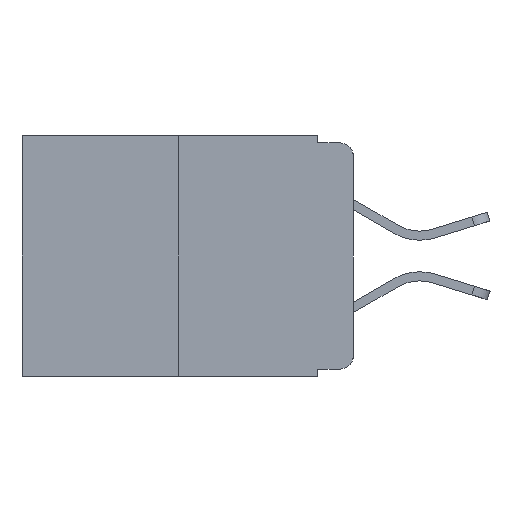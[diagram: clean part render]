
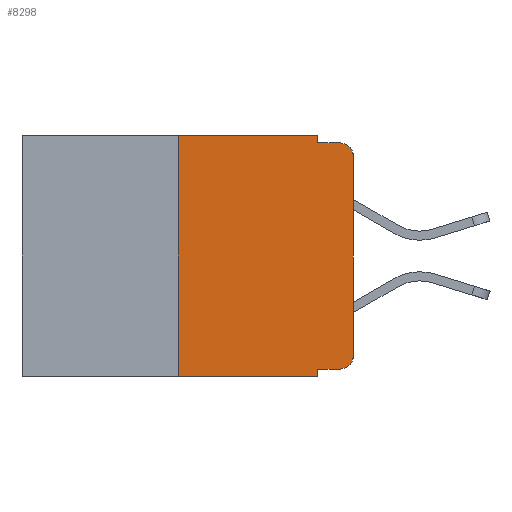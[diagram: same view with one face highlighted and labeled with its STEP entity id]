
A CAD part, left-side view. The second image highlights one B-rep face of the part: STEP entity #8298.
In plain terms, the highlighted planar face has unit normal (-1, 0, 0).
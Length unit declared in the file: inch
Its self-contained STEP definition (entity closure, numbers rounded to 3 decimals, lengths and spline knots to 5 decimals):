
#426 = EDGE_CURVE ( 'NONE', #20141, #12894, #7068, .T. ) ;
#635 = CARTESIAN_POINT ( 'NONE',  ( 0., 0., -0.313 ) ) ;
#849 = LINE ( 'NONE', #15361, #4133 ) ;
#969 = VECTOR ( 'NONE', #13384, 39.37008 ) ;
#1814 = CARTESIAN_POINT ( 'NONE',  ( 0., 0.25, -0.343 ) ) ;
#1913 = EDGE_CURVE ( 'NONE', #13388, #16300, #17655, .T. ) ;
#1970 = CARTESIAN_POINT ( 'NONE',  ( 0., 0.02, -0.313 ) ) ;
#2210 = VERTEX_POINT ( 'NONE', #3482 ) ;
#2233 = VECTOR ( 'NONE', #20647, 39.37008 ) ;
#2246 = LINE ( 'NONE', #18679, #21154 ) ;
#2588 = LINE ( 'NONE', #6047, #2233 ) ;
#2892 = ORIENTED_EDGE ( 'NONE', *, *, #12941, .T. ) ;
#3252 = PLANE ( 'NONE',  #8954 ) ;
#3482 = CARTESIAN_POINT ( 'NONE',  ( 0., 0., -0.03 ) ) ;
#3603 = CARTESIAN_POINT ( 'NONE',  ( 0., 0.051, -0.333 ) ) ;
#4133 = VECTOR ( 'NONE', #9190, 39.37008 ) ;
#4142 = CARTESIAN_POINT ( 'NONE',  ( 0., 0.051, -0.333 ) ) ;
#4661 = DIRECTION ( 'NONE',  ( 0., 0., -1. ) ) ;
#4762 = DIRECTION ( 'NONE',  ( 1., 0., 0. ) ) ;
#4946 = CARTESIAN_POINT ( 'NONE',  ( 0., 0.02, -0.333 ) ) ;
#5320 = EDGE_CURVE ( 'NONE', #16300, #13942, #5418, .T. ) ;
#5418 = CIRCLE ( 'NONE', #11596, 0.02 ) ;
#5475 = LINE ( 'NONE', #12148, #11381 ) ;
#5669 = ORIENTED_EDGE ( 'NONE', *, *, #7285, .F. ) ;
#6047 = CARTESIAN_POINT ( 'NONE',  ( 0., 0.051, 0. ) ) ;
#6206 = VERTEX_POINT ( 'NONE', #10444 ) ;
#7068 = LINE ( 'NONE', #18531, #14576 ) ;
#7285 = EDGE_CURVE ( 'NONE', #12894, #18009, #8433, .T. ) ;
#7309 = LINE ( 'NONE', #20509, #10439 ) ;
#8298 = ADVANCED_FACE ( 'NONE', ( #9939 ), #3252, .F. ) ;
#8433 = LINE ( 'NONE', #15023, #969 ) ;
#8557 = DIRECTION ( 'NONE',  ( -1., 0., 0. ) ) ;
#8756 = DIRECTION ( 'NONE',  ( 0., 0., -1. ) ) ;
#8811 = CARTESIAN_POINT ( 'NONE',  ( 0., 0.25, 0. ) ) ;
#8875 = DIRECTION ( 'NONE',  ( 0., 0., -1. ) ) ;
#8903 = ORIENTED_EDGE ( 'NONE', *, *, #16591, .F. ) ;
#8954 = AXIS2_PLACEMENT_3D ( 'NONE', #19467, #4762, #4661 ) ;
#9152 = DIRECTION ( 'NONE',  ( 0., 0., -1. ) ) ;
#9190 = DIRECTION ( 'NONE',  ( 0., -1., 0. ) ) ;
#9584 = ORIENTED_EDGE ( 'NONE', *, *, #21218, .F. ) ;
#9939 = FACE_OUTER_BOUND ( 'NONE', #19172, .T. ) ;
#10002 = DIRECTION ( 'NONE',  ( 0., 0., 1. ) ) ;
#10439 = VECTOR ( 'NONE', #9152, 39.37008 ) ;
#10444 = CARTESIAN_POINT ( 'NONE',  ( 0., 0.02, -0.01 ) ) ;
#10720 = DIRECTION ( 'NONE',  ( 0., -1., 0. ) ) ;
#11090 = ORIENTED_EDGE ( 'NONE', *, *, #12618, .T. ) ;
#11381 = VECTOR ( 'NONE', #10002, 39.37008 ) ;
#11596 = AXIS2_PLACEMENT_3D ( 'NONE', #1970, #8557, #8875 ) ;
#11805 = VECTOR ( 'NONE', #10720, 39.37008 ) ;
#11954 = DIRECTION ( 'NONE',  ( 0., -1., 0. ) ) ;
#12009 = CARTESIAN_POINT ( 'NONE',  ( 0., 0.051, -0.01 ) ) ;
#12052 = ORIENTED_EDGE ( 'NONE', *, *, #5320, .T. ) ;
#12148 = CARTESIAN_POINT ( 'NONE',  ( 0., 0., 0. ) ) ;
#12618 = EDGE_CURVE ( 'NONE', #2210, #6206, #16963, .T. ) ;
#12894 = VERTEX_POINT ( 'NONE', #8811 ) ;
#12941 = EDGE_CURVE ( 'NONE', #13942, #2210, #5475, .T. ) ;
#13384 = DIRECTION ( 'NONE',  ( 0., -1., 0. ) ) ;
#13388 = VERTEX_POINT ( 'NONE', #3603 ) ;
#13827 = AXIS2_PLACEMENT_3D ( 'NONE', #15566, #17305, #8756 ) ;
#13883 = ORIENTED_EDGE ( 'NONE', *, *, #13978, .F. ) ;
#13942 = VERTEX_POINT ( 'NONE', #635 ) ;
#13978 = EDGE_CURVE ( 'NONE', #18672, #6206, #849, .T. ) ;
#14429 = VERTEX_POINT ( 'NONE', #20840 ) ;
#14576 = VECTOR ( 'NONE', #15276, 39.37008 ) ;
#15023 = CARTESIAN_POINT ( 'NONE',  ( 0., 0.473, 0. ) ) ;
#15276 = DIRECTION ( 'NONE',  ( 0., 0., 1. ) ) ;
#15361 = CARTESIAN_POINT ( 'NONE',  ( 0., 0.051, -0.01 ) ) ;
#15566 = CARTESIAN_POINT ( 'NONE',  ( 0., 0.02, -0.03 ) ) ;
#16300 = VERTEX_POINT ( 'NONE', #4946 ) ;
#16591 = EDGE_CURVE ( 'NONE', #13388, #14429, #7309, .T. ) ;
#16608 = ORIENTED_EDGE ( 'NONE', *, *, #19137, .T. ) ;
#16963 = CIRCLE ( 'NONE', #13827, 0.02 ) ;
#17305 = DIRECTION ( 'NONE',  ( -1., 0., 0. ) ) ;
#17655 = LINE ( 'NONE', #4142, #11805 ) ;
#17805 = CARTESIAN_POINT ( 'NONE',  ( 0., 0.051, 0. ) ) ;
#18009 = VERTEX_POINT ( 'NONE', #17805 ) ;
#18343 = ORIENTED_EDGE ( 'NONE', *, *, #426, .F. ) ;
#18531 = CARTESIAN_POINT ( 'NONE',  ( 0., 0.25, 0. ) ) ;
#18672 = VERTEX_POINT ( 'NONE', #12009 ) ;
#18679 = CARTESIAN_POINT ( 'NONE',  ( 0., 0.473, -0.343 ) ) ;
#18686 = ORIENTED_EDGE ( 'NONE', *, *, #1913, .T. ) ;
#19137 = EDGE_CURVE ( 'NONE', #20141, #14429, #2246, .T. ) ;
#19172 = EDGE_LOOP ( 'NONE', ( #2892, #11090, #13883, #9584, #5669, #18343, #16608, #8903, #18686, #12052 ) ) ;
#19467 = CARTESIAN_POINT ( 'NONE',  ( 0., 0.473, 0. ) ) ;
#20141 = VERTEX_POINT ( 'NONE', #1814 ) ;
#20509 = CARTESIAN_POINT ( 'NONE',  ( 0., 0.051, 0. ) ) ;
#20647 = DIRECTION ( 'NONE',  ( 0., 0., -1. ) ) ;
#20840 = CARTESIAN_POINT ( 'NONE',  ( 0., 0.051, -0.343 ) ) ;
#21154 = VECTOR ( 'NONE', #11954, 39.37008 ) ;
#21218 = EDGE_CURVE ( 'NONE', #18009, #18672, #2588, .T. ) ;
